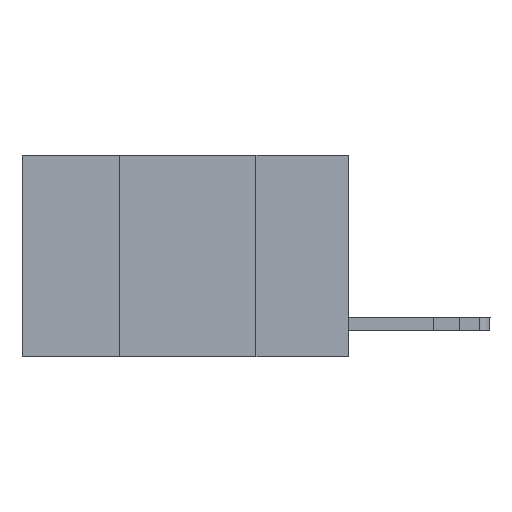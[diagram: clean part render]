
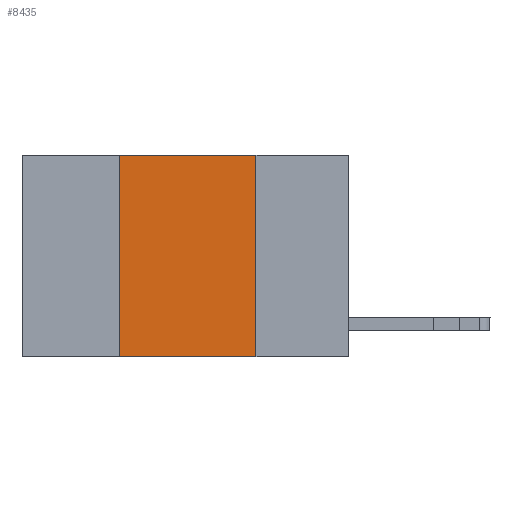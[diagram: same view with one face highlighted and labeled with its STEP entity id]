
A CAD part, left-side view. The second image highlights one B-rep face of the part: STEP entity #8435.
In plain terms, the highlighted planar face has unit normal (-1, 0, 0).
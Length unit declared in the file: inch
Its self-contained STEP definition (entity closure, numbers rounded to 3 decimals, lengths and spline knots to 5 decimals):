
#1059 = CARTESIAN_POINT ( 'NONE',  ( 0., 0.42, 0. ) ) ;
#1216 = CARTESIAN_POINT ( 'NONE',  ( 0., 0.17, 0. ) ) ;
#1293 = DIRECTION ( 'NONE',  ( 0., -1., 0. ) ) ;
#2427 = CARTESIAN_POINT ( 'NONE',  ( 0., 0.17, 0. ) ) ;
#2982 = DIRECTION ( 'NONE',  ( 1., 0., 0. ) ) ;
#3098 = VECTOR ( 'NONE', #1293, 39.37008 ) ;
#3629 = VERTEX_POINT ( 'NONE', #9102 ) ;
#3708 = ORIENTED_EDGE ( 'NONE', *, *, #19003, .F. ) ;
#5061 = PLANE ( 'NONE',  #17293 ) ;
#5880 = VERTEX_POINT ( 'NONE', #21086 ) ;
#8392 = VECTOR ( 'NONE', #22929, 39.37008 ) ;
#8435 = ADVANCED_FACE ( 'NONE', ( #14083 ), #5061, .F. ) ;
#8785 = CARTESIAN_POINT ( 'NONE',  ( 0., 0.6, -0.37 ) ) ;
#9102 = CARTESIAN_POINT ( 'NONE',  ( 0., 0.42, -0.37 ) ) ;
#10028 = CARTESIAN_POINT ( 'NONE',  ( 0., 0.42, 0. ) ) ;
#10588 = ORIENTED_EDGE ( 'NONE', *, *, #13503, .T. ) ;
#10767 = VERTEX_POINT ( 'NONE', #1216 ) ;
#11160 = VECTOR ( 'NONE', #18937, 39.37008 ) ;
#11740 = CARTESIAN_POINT ( 'NONE',  ( 0., 0.6, 0. ) ) ;
#13356 = CARTESIAN_POINT ( 'NONE',  ( 0., 0.6, 0. ) ) ;
#13503 = EDGE_CURVE ( 'NONE', #3629, #5880, #23920, .T. ) ;
#14083 = FACE_OUTER_BOUND ( 'NONE', #18287, .T. ) ;
#14146 = LINE ( 'NONE', #11740, #3098 ) ;
#15346 = LINE ( 'NONE', #1059, #15998 ) ;
#15998 = VECTOR ( 'NONE', #17616, 39.37008 ) ;
#17188 = LINE ( 'NONE', #2427, #11160 ) ;
#17293 = AXIS2_PLACEMENT_3D ( 'NONE', #13356, #2982, #17440 ) ;
#17440 = DIRECTION ( 'NONE',  ( 0., 0., -1. ) ) ;
#17616 = DIRECTION ( 'NONE',  ( 0., 0., 1. ) ) ;
#18287 = EDGE_LOOP ( 'NONE', ( #24808, #3708, #20089, #10588 ) ) ;
#18937 = DIRECTION ( 'NONE',  ( 0., 0., -1. ) ) ;
#19003 = EDGE_CURVE ( 'NONE', #20881, #10767, #14146, .T. ) ;
#20089 = ORIENTED_EDGE ( 'NONE', *, *, #20288, .F. ) ;
#20288 = EDGE_CURVE ( 'NONE', #3629, #20881, #15346, .T. ) ;
#20881 = VERTEX_POINT ( 'NONE', #10028 ) ;
#21086 = CARTESIAN_POINT ( 'NONE',  ( 0., 0.17, -0.37 ) ) ;
#21132 = EDGE_CURVE ( 'NONE', #10767, #5880, #17188, .T. ) ;
#22929 = DIRECTION ( 'NONE',  ( 0., -1., 0. ) ) ;
#23920 = LINE ( 'NONE', #8785, #8392 ) ;
#24808 = ORIENTED_EDGE ( 'NONE', *, *, #21132, .F. ) ;
